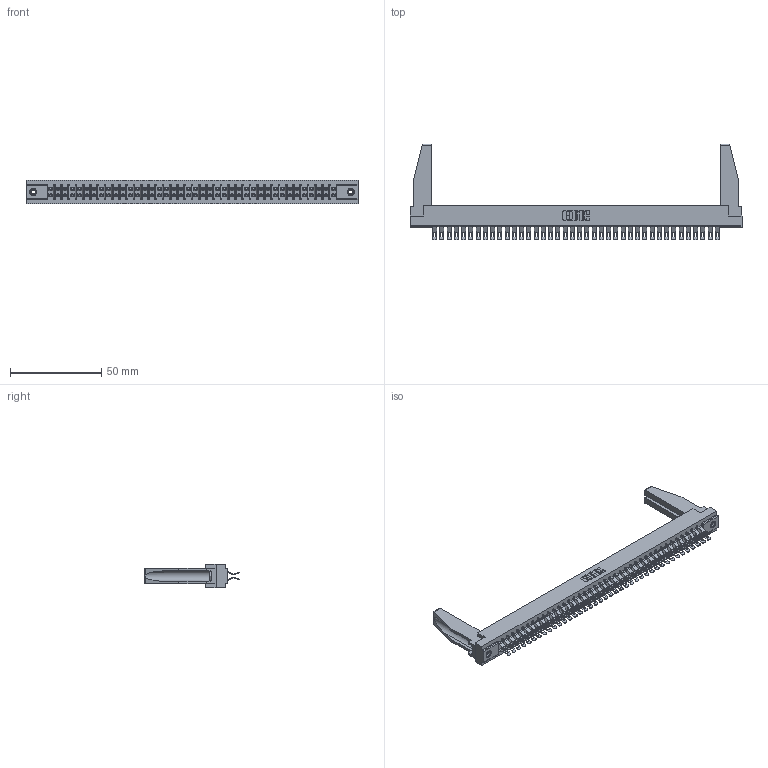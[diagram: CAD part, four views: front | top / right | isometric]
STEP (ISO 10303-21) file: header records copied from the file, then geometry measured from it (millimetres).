
FILE_DESCRIPTION (( 'STEP AP203' ), '1' );
FILE_NAME ('357-080-455-278.STEP', '2020-10-04T11:25:10', ( '' ), ( '' ), 'SwSTEP 2.0', 'SolidWorks 2020', '' );
FILE_SCHEMA (( 'CONFIG_CONTROL_DESIGN' ));
Length unit declared in the file: inch
Products named in the file (5): 307-220-078; 345-250-001_345-250-001-102; 307-290-001_555; 307 Part_.156 Dia Mounting Holes; 357-080-455-278
Assembly tree (85 placements, depth 2):
  357-080-455-278
    307 Part_.156 Dia Mounting Holes
    307-290-001_555  x80
    307-220-078  x2
    345-250-001_345-250-001-102  x2
Bounding box: 181.51 x 52.45 x 12.7 mm (x, y, z)
Volume: 23518.8 mm3; surface area: 28999.6 mm2
Topology: 85 solids, 85 shells, 5169 faces, 15133 edges, 9862 vertices
Faces by surface type: plane 2874, cylinder 2197, sphere 82, cone 12, torus 4
Entity records: 38794 total; most frequent: CARTESIAN_POINT 6362, ORIENTED_EDGE 6266, DIRECTION 6193, EDGE_CURVE 3133, VECTOR 2395, LINE 2395, VERTEX_POINT 2026, AXIS2_PLACEMENT_3D 1899
